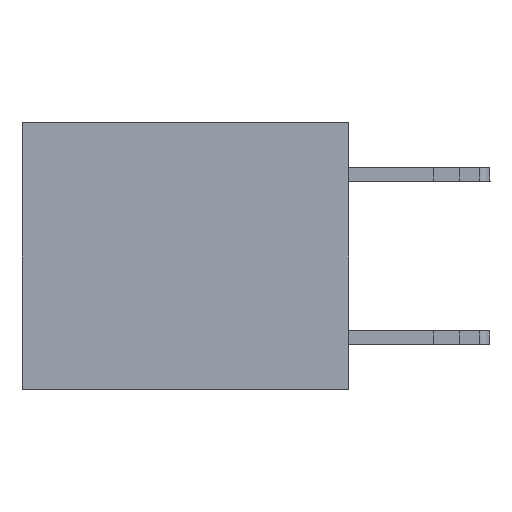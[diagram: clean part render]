
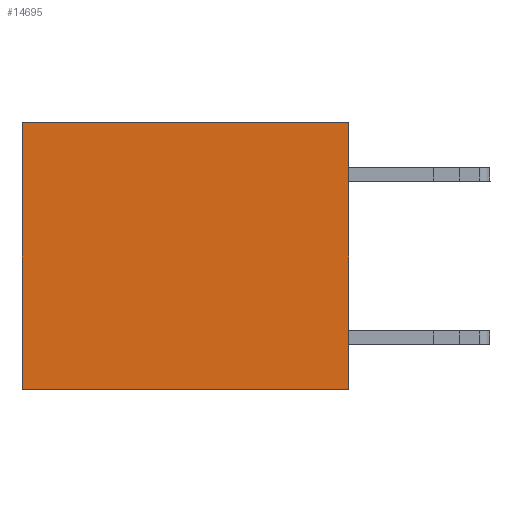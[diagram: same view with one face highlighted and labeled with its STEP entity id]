
A CAD part, left-side view. The second image highlights one B-rep face of the part: STEP entity #14695.
In plain terms, the highlighted planar face has unit normal (-1, 0, 0).
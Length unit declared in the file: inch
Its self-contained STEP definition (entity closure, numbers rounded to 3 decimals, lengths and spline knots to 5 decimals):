
#279 = VERTEX_POINT ( 'NONE', #25135 ) ;
#1905 = LINE ( 'NONE', #6173, #15546 ) ;
#2364 = DIRECTION ( 'NONE',  ( 0., 0., -1. ) ) ;
#3756 = DIRECTION ( 'NONE',  ( 0., 1., 0. ) ) ;
#4059 = CARTESIAN_POINT ( 'NONE',  ( 0.3165, 0.6, 0. ) ) ;
#4107 = ORIENTED_EDGE ( 'NONE', *, *, #4486, .F. ) ;
#4486 = EDGE_CURVE ( 'NONE', #23859, #279, #16558, .T. ) ;
#4508 = CARTESIAN_POINT ( 'NONE',  ( 0.3165, 0., 0. ) ) ;
#4651 = LINE ( 'NONE', #15189, #8545 ) ;
#6173 = CARTESIAN_POINT ( 'NONE',  ( 0.3165, 0.6, -0.49 ) ) ;
#6181 = ORIENTED_EDGE ( 'NONE', *, *, #20969, .T. ) ;
#8497 = CARTESIAN_POINT ( 'NONE',  ( 0.3165, 0.6, -0.49 ) ) ;
#8545 = VECTOR ( 'NONE', #3756, 39.37008 ) ;
#8928 = VECTOR ( 'NONE', #16318, 39.37008 ) ;
#9527 = ORIENTED_EDGE ( 'NONE', *, *, #13917, .F. ) ;
#10573 = DIRECTION ( 'NONE',  ( 0., 0., -1. ) ) ;
#11076 = EDGE_LOOP ( 'NONE', ( #6181, #9527, #4107, #13367 ) ) ;
#13097 = PLANE ( 'NONE',  #20168 ) ;
#13367 = ORIENTED_EDGE ( 'NONE', *, *, #18719, .T. ) ;
#13917 = EDGE_CURVE ( 'NONE', #279, #22094, #4651, .T. ) ;
#14695 = ADVANCED_FACE ( 'NONE', ( #22580 ), #13097, .F. ) ;
#15189 = CARTESIAN_POINT ( 'NONE',  ( 0.3165, 0., -0.49 ) ) ;
#15259 = CARTESIAN_POINT ( 'NONE',  ( 0.3165, 0., 0. ) ) ;
#15546 = VECTOR ( 'NONE', #2364, 39.37008 ) ;
#16318 = DIRECTION ( 'NONE',  ( 0., 1., 0. ) ) ;
#16558 = LINE ( 'NONE', #16571, #17774 ) ;
#16571 = CARTESIAN_POINT ( 'NONE',  ( 0.3165, 0., -0.49 ) ) ;
#16753 = DIRECTION ( 'NONE',  ( 0., 0., -1. ) ) ;
#17004 = CARTESIAN_POINT ( 'NONE',  ( 0.3165, 0., -0.49 ) ) ;
#17774 = VECTOR ( 'NONE', #10573, 39.37008 ) ;
#18719 = EDGE_CURVE ( 'NONE', #23859, #23772, #24792, .T. ) ;
#18960 = DIRECTION ( 'NONE',  ( 1., 0., 0. ) ) ;
#20168 = AXIS2_PLACEMENT_3D ( 'NONE', #17004, #18960, #16753 ) ;
#20969 = EDGE_CURVE ( 'NONE', #23772, #22094, #1905, .T. ) ;
#22094 = VERTEX_POINT ( 'NONE', #8497 ) ;
#22580 = FACE_OUTER_BOUND ( 'NONE', #11076, .T. ) ;
#23772 = VERTEX_POINT ( 'NONE', #4059 ) ;
#23859 = VERTEX_POINT ( 'NONE', #15259 ) ;
#24792 = LINE ( 'NONE', #4508, #8928 ) ;
#25135 = CARTESIAN_POINT ( 'NONE',  ( 0.3165, 0., -0.49 ) ) ;
